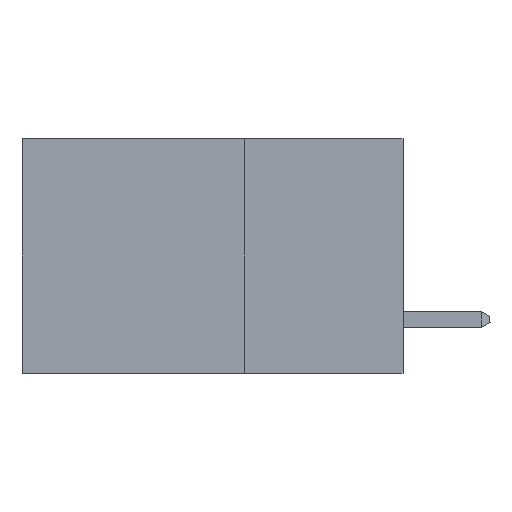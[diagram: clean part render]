
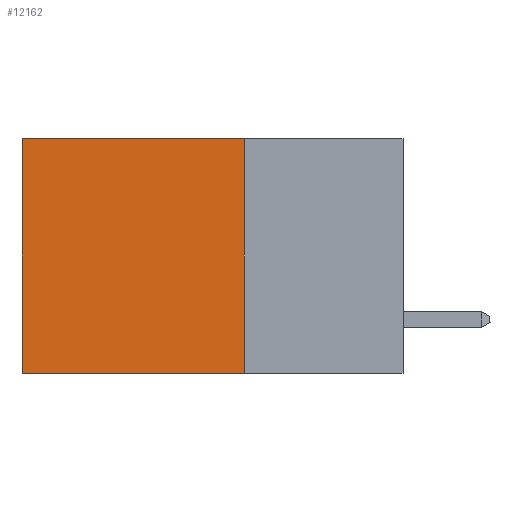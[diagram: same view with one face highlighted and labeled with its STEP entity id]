
A CAD part, left-side view. The second image highlights one B-rep face of the part: STEP entity #12162.
In plain terms, the highlighted planar face has unit normal (-1, 0, 0).
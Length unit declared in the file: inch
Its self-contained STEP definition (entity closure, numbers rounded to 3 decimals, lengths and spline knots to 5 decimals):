
#52 = ORIENTED_EDGE ( 'NONE', *, *, #36208, .F. ) ;
#462 = LINE ( 'NONE', #22202, #14561 ) ;
#904 = CARTESIAN_POINT ( 'NONE',  ( 0.2875, 0.25, 0. ) ) ;
#2002 = LINE ( 'NONE', #45459, #23653 ) ;
#2932 = CARTESIAN_POINT ( 'NONE',  ( 0.2875, 0.25, -0.37 ) ) ;
#8307 = DIRECTION ( 'NONE',  ( 0., 0., -1. ) ) ;
#8460 = LINE ( 'NONE', #32552, #16121 ) ;
#9726 = DIRECTION ( 'NONE',  ( 1., 0., 0. ) ) ;
#11348 = DIRECTION ( 'NONE',  ( 0., 1., 0. ) ) ;
#12162 = ADVANCED_FACE ( 'NONE', ( #25029 ), #24461, .F. ) ;
#14561 = VECTOR ( 'NONE', #11348, 39.37008 ) ;
#16121 = VECTOR ( 'NONE', #43649, 39.37008 ) ;
#16348 = VERTEX_POINT ( 'NONE', #2932 ) ;
#19054 = VERTEX_POINT ( 'NONE', #31020 ) ;
#22202 = CARTESIAN_POINT ( 'NONE',  ( 0.2875, 0.25, 0. ) ) ;
#22668 = CARTESIAN_POINT ( 'NONE',  ( 0.2875, 0.6, 0. ) ) ;
#23653 = VECTOR ( 'NONE', #8307, 39.37008 ) ;
#24113 = ORIENTED_EDGE ( 'NONE', *, *, #31527, .T. ) ;
#24461 = PLANE ( 'NONE',  #39399 ) ;
#24977 = VERTEX_POINT ( 'NONE', #904 ) ;
#25029 = FACE_OUTER_BOUND ( 'NONE', #36883, .T. ) ;
#28093 = ORIENTED_EDGE ( 'NONE', *, *, #40545, .T. ) ;
#31020 = CARTESIAN_POINT ( 'NONE',  ( 0.2875, 0.6, 0. ) ) ;
#31527 = EDGE_CURVE ( 'NONE', #24977, #19054, #462, .T. ) ;
#32221 = CARTESIAN_POINT ( 'NONE',  ( 0.2875, 0.25, 0. ) ) ;
#32542 = ORIENTED_EDGE ( 'NONE', *, *, #36798, .F. ) ;
#32552 = CARTESIAN_POINT ( 'NONE',  ( 0.2875, 0.25, -0.37 ) ) ;
#33090 = VECTOR ( 'NONE', #40568, 39.37008 ) ;
#34316 = CARTESIAN_POINT ( 'NONE',  ( 0.2875, 0.6, -0.37 ) ) ;
#36208 = EDGE_CURVE ( 'NONE', #16348, #48130, #8460, .T. ) ;
#36798 = EDGE_CURVE ( 'NONE', #24977, #16348, #2002, .T. ) ;
#36883 = EDGE_LOOP ( 'NONE', ( #28093, #52, #32542, #24113 ) ) ;
#39399 = AXIS2_PLACEMENT_3D ( 'NONE', #32221, #9726, #42991 ) ;
#39579 = LINE ( 'NONE', #22668, #33090 ) ;
#40545 = EDGE_CURVE ( 'NONE', #19054, #48130, #39579, .T. ) ;
#40568 = DIRECTION ( 'NONE',  ( 0., 0., -1. ) ) ;
#42991 = DIRECTION ( 'NONE',  ( 0., 0., -1. ) ) ;
#43649 = DIRECTION ( 'NONE',  ( 0., 1., 0. ) ) ;
#45459 = CARTESIAN_POINT ( 'NONE',  ( 0.2875, 0.25, 0. ) ) ;
#48130 = VERTEX_POINT ( 'NONE', #34316 ) ;
